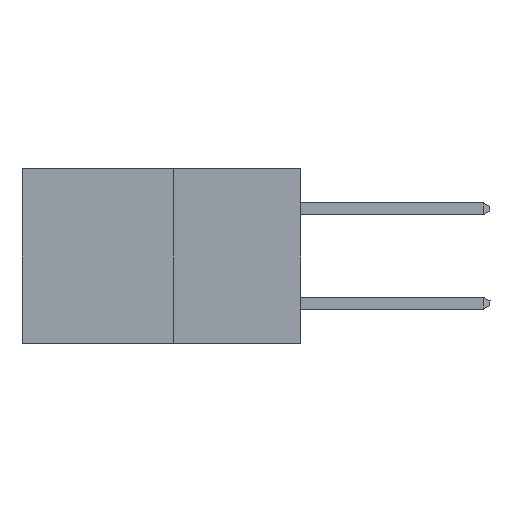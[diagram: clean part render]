
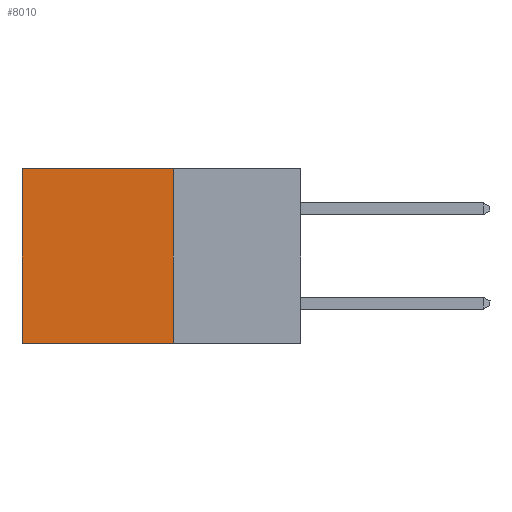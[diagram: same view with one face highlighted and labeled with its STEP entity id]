
A CAD part, left-side view. The second image highlights one B-rep face of the part: STEP entity #8010.
In plain terms, the highlighted planar face has unit normal (-1, 0, 0).
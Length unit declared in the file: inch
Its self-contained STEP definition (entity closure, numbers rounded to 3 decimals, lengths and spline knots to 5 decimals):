
#1957 = EDGE_LOOP ( 'NONE', ( #30778, #17288, #13377, #31132 ) ) ;
#2425 = DIRECTION ( 'NONE',  ( 0., 0., -1. ) ) ;
#2537 = DIRECTION ( 'NONE',  ( 1., 0., 0. ) ) ;
#2861 = PLANE ( 'NONE',  #20982 ) ;
#3834 = VERTEX_POINT ( 'NONE', #27972 ) ;
#4630 = DIRECTION ( 'NONE',  ( 0., 1., 0. ) ) ;
#4880 = CARTESIAN_POINT ( 'NONE',  ( 0.277, 0.27, -0.37 ) ) ;
#4892 = EDGE_CURVE ( 'NONE', #3834, #24154, #31473, .T. ) ;
#5162 = VECTOR ( 'NONE', #30073, 39.37008 ) ;
#5239 = CARTESIAN_POINT ( 'NONE',  ( 0.277, 0.27, 0. ) ) ;
#8010 = ADVANCED_FACE ( 'NONE', ( #21823 ), #2861, .F. ) ;
#9633 = CARTESIAN_POINT ( 'NONE',  ( 0.277, 0.27, -0.37 ) ) ;
#9741 = CARTESIAN_POINT ( 'NONE',  ( 0.277, 0.27, -0.37 ) ) ;
#11807 = VECTOR ( 'NONE', #4630, 39.37008 ) ;
#13377 = ORIENTED_EDGE ( 'NONE', *, *, #4892, .F. ) ;
#14267 = VERTEX_POINT ( 'NONE', #31334 ) ;
#15544 = EDGE_CURVE ( 'NONE', #3834, #27916, #25204, .T. ) ;
#16896 = LINE ( 'NONE', #9741, #11807 ) ;
#17288 = ORIENTED_EDGE ( 'NONE', *, *, #21487, .F. ) ;
#20773 = LINE ( 'NONE', #22192, #27177 ) ;
#20982 = AXIS2_PLACEMENT_3D ( 'NONE', #4880, #2537, #2425 ) ;
#21487 = EDGE_CURVE ( 'NONE', #24154, #14267, #16896, .T. ) ;
#21823 = FACE_OUTER_BOUND ( 'NONE', #1957, .T. ) ;
#22192 = CARTESIAN_POINT ( 'NONE',  ( 0.277, 0.59, -0.37 ) ) ;
#22658 = DIRECTION ( 'NONE',  ( 0., 1., 0. ) ) ;
#24154 = VERTEX_POINT ( 'NONE', #9633 ) ;
#24441 = VECTOR ( 'NONE', #22658, 39.37008 ) ;
#24570 = CARTESIAN_POINT ( 'NONE',  ( 0.277, 0.59, 0. ) ) ;
#24602 = DIRECTION ( 'NONE',  ( 0., 0., -1. ) ) ;
#25204 = LINE ( 'NONE', #5239, #24441 ) ;
#26234 = EDGE_CURVE ( 'NONE', #27916, #14267, #20773, .T. ) ;
#27177 = VECTOR ( 'NONE', #24602, 39.37008 ) ;
#27916 = VERTEX_POINT ( 'NONE', #24570 ) ;
#27972 = CARTESIAN_POINT ( 'NONE',  ( 0.277, 0.27, 0. ) ) ;
#30073 = DIRECTION ( 'NONE',  ( 0., 0., -1. ) ) ;
#30371 = CARTESIAN_POINT ( 'NONE',  ( 0.277, 0.27, -0.37 ) ) ;
#30778 = ORIENTED_EDGE ( 'NONE', *, *, #26234, .T. ) ;
#31132 = ORIENTED_EDGE ( 'NONE', *, *, #15544, .T. ) ;
#31334 = CARTESIAN_POINT ( 'NONE',  ( 0.277, 0.59, -0.37 ) ) ;
#31473 = LINE ( 'NONE', #30371, #5162 ) ;
